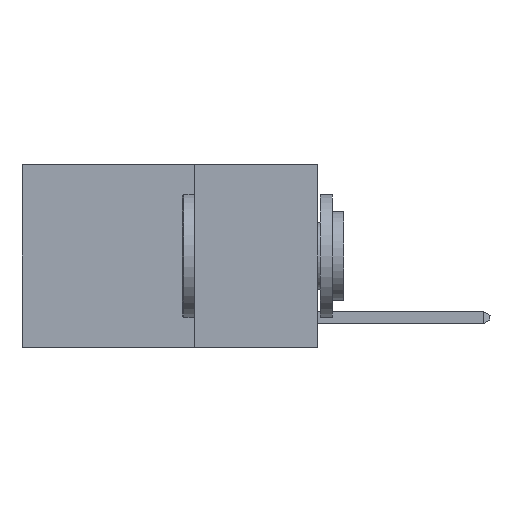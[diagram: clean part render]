
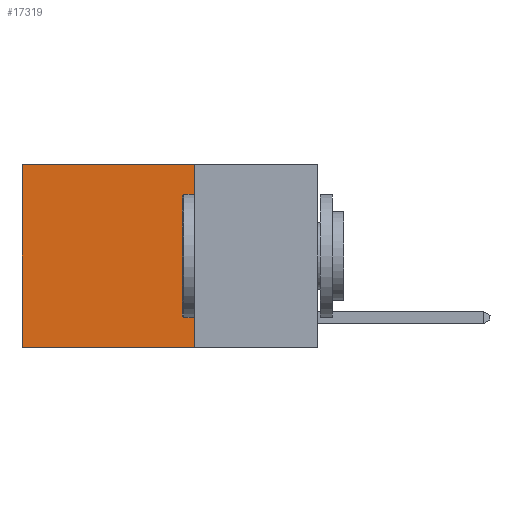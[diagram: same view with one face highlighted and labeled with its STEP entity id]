
A CAD part, left-side view. The second image highlights one B-rep face of the part: STEP entity #17319.
In plain terms, the highlighted planar face has unit normal (-1, 0, 0).
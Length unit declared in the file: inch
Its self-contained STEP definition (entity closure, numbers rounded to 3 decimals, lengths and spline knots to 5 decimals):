
#1160 = CARTESIAN_POINT ( 'NONE',  ( 0.2625, 0.6, 0. ) ) ;
#1864 = CARTESIAN_POINT ( 'NONE',  ( 0.2625, 0.25, -0.37 ) ) ;
#2111 = CARTESIAN_POINT ( 'NONE',  ( 0.2625, 0.6, 0. ) ) ;
#2154 = EDGE_LOOP ( 'NONE', ( #17242, #18721, #15285, #20543 ) ) ;
#2319 = PLANE ( 'NONE',  #10692 ) ;
#2430 = CARTESIAN_POINT ( 'NONE',  ( 0.2625, 0.25, 0. ) ) ;
#3061 = DIRECTION ( 'NONE',  ( 0., 1., 0. ) ) ;
#3415 = VERTEX_POINT ( 'NONE', #2111 ) ;
#3629 = EDGE_CURVE ( 'NONE', #9121, #3415, #3921, .T. ) ;
#3921 = LINE ( 'NONE', #7145, #4397 ) ;
#4397 = VECTOR ( 'NONE', #19065, 39.37008 ) ;
#6090 = LINE ( 'NONE', #1160, #16571 ) ;
#7145 = CARTESIAN_POINT ( 'NONE',  ( 0.2625, 0.25, 0. ) ) ;
#7731 = DIRECTION ( 'NONE',  ( 0., 0., -1. ) ) ;
#7938 = EDGE_CURVE ( 'NONE', #9905, #8775, #12920, .T. ) ;
#8022 = CARTESIAN_POINT ( 'NONE',  ( 0.2625, 0.25, -0.37 ) ) ;
#8775 = VERTEX_POINT ( 'NONE', #15311 ) ;
#9093 = CARTESIAN_POINT ( 'NONE',  ( 0.2625, 0.25, 0. ) ) ;
#9121 = VERTEX_POINT ( 'NONE', #2430 ) ;
#9905 = VERTEX_POINT ( 'NONE', #1864 ) ;
#10692 = AXIS2_PLACEMENT_3D ( 'NONE', #12271, #17436, #17224 ) ;
#10831 = EDGE_CURVE ( 'NONE', #9121, #9905, #19054, .T. ) ;
#10848 = FACE_OUTER_BOUND ( 'NONE', #2154, .T. ) ;
#12040 = DIRECTION ( 'NONE',  ( 0., 0., -1. ) ) ;
#12271 = CARTESIAN_POINT ( 'NONE',  ( 0.2625, 0.25, 0. ) ) ;
#12920 = LINE ( 'NONE', #8022, #20694 ) ;
#15113 = VECTOR ( 'NONE', #12040, 39.37008 ) ;
#15285 = ORIENTED_EDGE ( 'NONE', *, *, #10831, .F. ) ;
#15311 = CARTESIAN_POINT ( 'NONE',  ( 0.2625, 0.6, -0.37 ) ) ;
#16571 = VECTOR ( 'NONE', #7731, 39.37008 ) ;
#17224 = DIRECTION ( 'NONE',  ( 0., 0., -1. ) ) ;
#17242 = ORIENTED_EDGE ( 'NONE', *, *, #18162, .T. ) ;
#17319 = ADVANCED_FACE ( 'NONE', ( #10848 ), #2319, .F. ) ;
#17436 = DIRECTION ( 'NONE',  ( 1., 0., 0. ) ) ;
#18162 = EDGE_CURVE ( 'NONE', #3415, #8775, #6090, .T. ) ;
#18721 = ORIENTED_EDGE ( 'NONE', *, *, #7938, .F. ) ;
#19054 = LINE ( 'NONE', #9093, #15113 ) ;
#19065 = DIRECTION ( 'NONE',  ( 0., 1., 0. ) ) ;
#20543 = ORIENTED_EDGE ( 'NONE', *, *, #3629, .T. ) ;
#20694 = VECTOR ( 'NONE', #3061, 39.37008 ) ;
